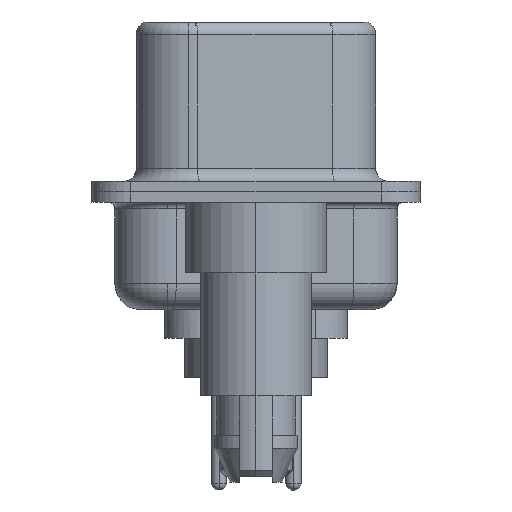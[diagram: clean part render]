
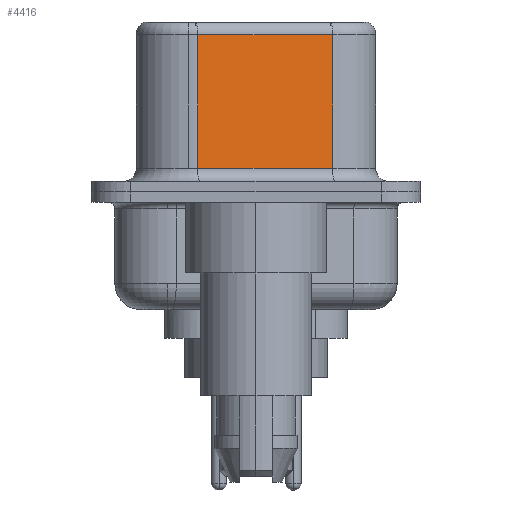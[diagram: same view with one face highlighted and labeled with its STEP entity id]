
A CAD part, left-side view. The second image highlights one B-rep face of the part: STEP entity #4416.
In plain terms, the highlighted planar face has unit normal (-0.985, -0.174, 0).
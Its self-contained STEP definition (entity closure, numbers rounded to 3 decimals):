
#198 = CARTESIAN_POINT ( 'NONE',  ( 4.58, -2.927, 0.9 ) ) ;
#480 = EDGE_CURVE ( 'NONE', #4392, #4202, #14245, .T. ) ;
#1476 = DIRECTION ( 'NONE',  ( 0.985, 0.174, 0. ) ) ;
#1629 = ORIENTED_EDGE ( 'NONE', *, *, #7088, .T. ) ;
#2249 = DIRECTION ( 'NONE',  ( 0., 0., -1. ) ) ;
#2655 = CARTESIAN_POINT ( 'NONE',  ( 3.67, 2.233, 0.9 ) ) ;
#2680 = DIRECTION ( 'NONE',  ( 0., 0., -1. ) ) ;
#2711 = EDGE_CURVE ( 'NONE', #7383, #4392, #19558, .T. ) ;
#2791 = LINE ( 'NONE', #7353, #14647 ) ;
#2851 = EDGE_LOOP ( 'NONE', ( #14710, #8063, #4369, #1629 ) ) ;
#3259 = PLANE ( 'NONE',  #17782 ) ;
#3333 = DIRECTION ( 'NONE',  ( 0.174, -0.985, 0. ) ) ;
#3806 = CARTESIAN_POINT ( 'NONE',  ( 4.58, -2.927, 6.52 ) ) ;
#4202 = VERTEX_POINT ( 'NONE', #2655 ) ;
#4369 = ORIENTED_EDGE ( 'NONE', *, *, #480, .T. ) ;
#4392 = VERTEX_POINT ( 'NONE', #11235 ) ;
#4407 = VERTEX_POINT ( 'NONE', #198 ) ;
#4416 = ADVANCED_FACE ( 'NONE', ( #5130 ), #3259, .F. ) ;
#5130 = FACE_OUTER_BOUND ( 'NONE', #2851, .T. ) ;
#7088 = EDGE_CURVE ( 'NONE', #4202, #4407, #13440, .T. ) ;
#7353 = CARTESIAN_POINT ( 'NONE',  ( 4.58, -2.927, 6.52 ) ) ;
#7383 = VERTEX_POINT ( 'NONE', #9614 ) ;
#8063 = ORIENTED_EDGE ( 'NONE', *, *, #2711, .T. ) ;
#9614 = CARTESIAN_POINT ( 'NONE',  ( 4.58, -2.927, 6.02 ) ) ;
#10229 = VECTOR ( 'NONE', #2249, 1000. ) ;
#10279 = CARTESIAN_POINT ( 'NONE',  ( 4.58, -2.927, 6.02 ) ) ;
#11235 = CARTESIAN_POINT ( 'NONE',  ( 3.67, 2.233, 6.02 ) ) ;
#11795 = VECTOR ( 'NONE', #12075, 1000. ) ;
#12075 = DIRECTION ( 'NONE',  ( -0.174, 0.985, 0. ) ) ;
#13440 = LINE ( 'NONE', #19132, #16560 ) ;
#14245 = LINE ( 'NONE', #14374, #10229 ) ;
#14374 = CARTESIAN_POINT ( 'NONE',  ( 3.67, 2.233, 6.52 ) ) ;
#14647 = VECTOR ( 'NONE', #2680, 1000. ) ;
#14710 = ORIENTED_EDGE ( 'NONE', *, *, #16907, .F. ) ;
#16560 = VECTOR ( 'NONE', #3333, 1000. ) ;
#16907 = EDGE_CURVE ( 'NONE', #7383, #4407, #2791, .T. ) ;
#17444 = DIRECTION ( 'NONE',  ( -0.174, 0.985, 0. ) ) ;
#17782 = AXIS2_PLACEMENT_3D ( 'NONE', #3806, #1476, #17444 ) ;
#19132 = CARTESIAN_POINT ( 'NONE',  ( 4.58, -2.927, 0.9 ) ) ;
#19558 = LINE ( 'NONE', #10279, #11795 ) ;
